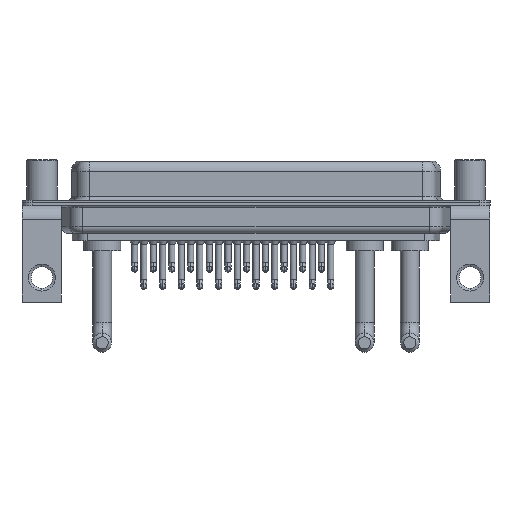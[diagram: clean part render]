
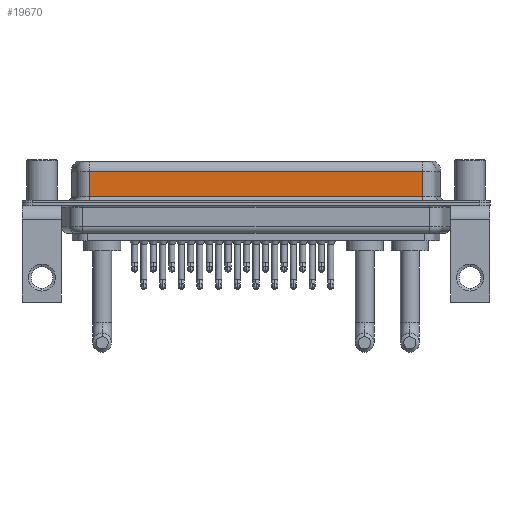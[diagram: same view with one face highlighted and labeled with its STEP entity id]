
A CAD part, front view. The second image highlights one B-rep face of the part: STEP entity #19670.
In plain terms, the highlighted planar face has unit normal (0, -1, 0).
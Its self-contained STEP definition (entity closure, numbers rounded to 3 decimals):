
#1089 = EDGE_CURVE ( 'NONE', #17468, #24209, #24685, .T. ) ;
#1459 = DIRECTION ( 'NONE',  ( 0., 0., -1. ) ) ;
#1562 = DIRECTION ( 'NONE',  ( 1., 0., 0. ) ) ;
#2380 = VECTOR ( 'NONE', #23614, 1000. ) ;
#2384 = CARTESIAN_POINT ( 'NONE',  ( 56.462, -3.95, 0.9 ) ) ;
#2687 = VECTOR ( 'NONE', #14704, 1000. ) ;
#3388 = EDGE_CURVE ( 'NONE', #17468, #6818, #9641, .T. ) ;
#3630 = EDGE_LOOP ( 'NONE', ( #18531, #25002, #4821, #15888 ) ) ;
#4081 = DIRECTION ( 'NONE',  ( 0., 0., 1. ) ) ;
#4821 = ORIENTED_EDGE ( 'NONE', *, *, #10712, .T. ) ;
#5978 = CARTESIAN_POINT ( 'NONE',  ( 7.038, -3.95, 6.4 ) ) ;
#6818 = VERTEX_POINT ( 'NONE', #9327 ) ;
#8675 = CARTESIAN_POINT ( 'NONE',  ( 7.038, -3.95, 0.9 ) ) ;
#9064 = VECTOR ( 'NONE', #1562, 1000. ) ;
#9327 = CARTESIAN_POINT ( 'NONE',  ( 7.038, -3.95, 4.65 ) ) ;
#9641 = LINE ( 'NONE', #15493, #2380 ) ;
#10712 = EDGE_CURVE ( 'NONE', #6818, #12765, #21688, .T. ) ;
#12765 = VERTEX_POINT ( 'NONE', #8675 ) ;
#13930 = DIRECTION ( 'NONE',  ( 0., 1., 0. ) ) ;
#14194 = FACE_OUTER_BOUND ( 'NONE', #3630, .T. ) ;
#14704 = DIRECTION ( 'NONE',  ( 0., 0., -1. ) ) ;
#15493 = CARTESIAN_POINT ( 'NONE',  ( 56.462, -3.95, 4.65 ) ) ;
#15888 = ORIENTED_EDGE ( 'NONE', *, *, #26307, .T. ) ;
#16075 = VECTOR ( 'NONE', #1459, 1000. ) ;
#16817 = CARTESIAN_POINT ( 'NONE',  ( 56.462, -3.95, 4.65 ) ) ;
#17468 = VERTEX_POINT ( 'NONE', #16817 ) ;
#17779 = PLANE ( 'NONE',  #25744 ) ;
#18423 = CARTESIAN_POINT ( 'NONE',  ( 56.462, -3.95, 6.4 ) ) ;
#18531 = ORIENTED_EDGE ( 'NONE', *, *, #1089, .F. ) ;
#19670 = ADVANCED_FACE ( 'NONE', ( #14194 ), #17779, .F. ) ;
#21688 = LINE ( 'NONE', #5978, #16075 ) ;
#23520 = CARTESIAN_POINT ( 'NONE',  ( 56.462, -3.95, 0.9 ) ) ;
#23614 = DIRECTION ( 'NONE',  ( -1., 0., 0. ) ) ;
#24209 = VERTEX_POINT ( 'NONE', #2384 ) ;
#24685 = LINE ( 'NONE', #18423, #2687 ) ;
#25002 = ORIENTED_EDGE ( 'NONE', *, *, #3388, .T. ) ;
#25744 = AXIS2_PLACEMENT_3D ( 'NONE', #26296, #13930, #4081 ) ;
#25910 = LINE ( 'NONE', #23520, #9064 ) ;
#26296 = CARTESIAN_POINT ( 'NONE',  ( 56.462, -3.95, 6.4 ) ) ;
#26307 = EDGE_CURVE ( 'NONE', #12765, #24209, #25910, .T. ) ;
